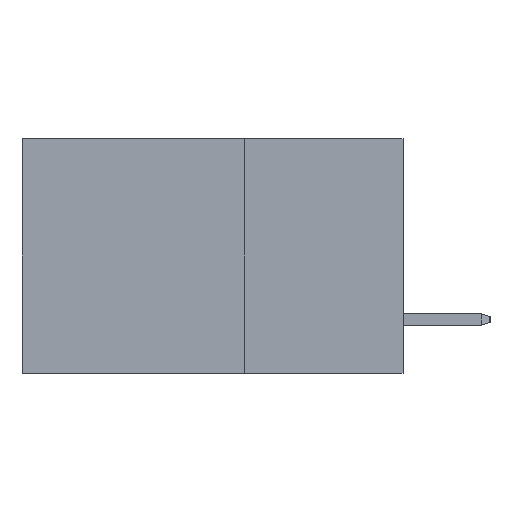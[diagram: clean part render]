
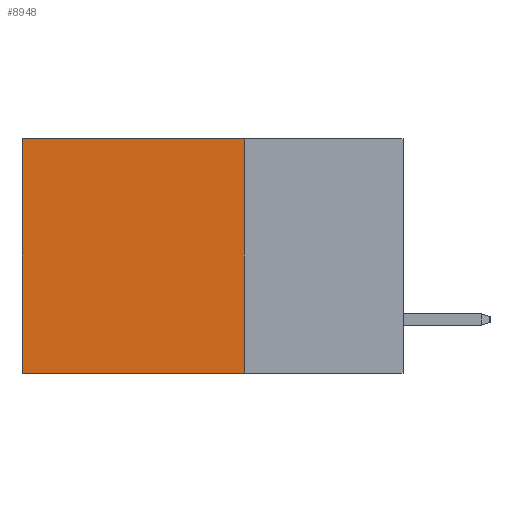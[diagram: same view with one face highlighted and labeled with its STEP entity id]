
A CAD part, left-side view. The second image highlights one B-rep face of the part: STEP entity #8948.
In plain terms, the highlighted planar face has unit normal (-1, 0, 0).
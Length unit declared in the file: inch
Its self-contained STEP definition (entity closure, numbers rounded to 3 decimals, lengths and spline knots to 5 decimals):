
#58 = PLANE ( 'NONE',  #7487 ) ;
#1327 = EDGE_LOOP ( 'NONE', ( #10557, #2436, #4083, #4589 ) ) ;
#2436 = ORIENTED_EDGE ( 'NONE', *, *, #5455, .F. ) ;
#2634 = CARTESIAN_POINT ( 'NONE',  ( 0.2875, 0.25, 0. ) ) ;
#2853 = CARTESIAN_POINT ( 'NONE',  ( 0.2875, 0.25, 0. ) ) ;
#3242 = DIRECTION ( 'NONE',  ( 0., 0., -1. ) ) ;
#3388 = DIRECTION ( 'NONE',  ( 0., 0., -1. ) ) ;
#3649 = VECTOR ( 'NONE', #3388, 39.37008 ) ;
#3777 = VERTEX_POINT ( 'NONE', #8731 ) ;
#4083 = ORIENTED_EDGE ( 'NONE', *, *, #8963, .F. ) ;
#4140 = CARTESIAN_POINT ( 'NONE',  ( 0.2875, 0.25, 0. ) ) ;
#4499 = VECTOR ( 'NONE', #8467, 39.37008 ) ;
#4589 = ORIENTED_EDGE ( 'NONE', *, *, #8456, .T. ) ;
#5147 = FACE_OUTER_BOUND ( 'NONE', #1327, .T. ) ;
#5455 = EDGE_CURVE ( 'NONE', #6212, #3777, #8843, .T. ) ;
#5502 = CARTESIAN_POINT ( 'NONE',  ( 0.2875, 0.6, 0. ) ) ;
#6212 = VERTEX_POINT ( 'NONE', #12421 ) ;
#6459 = DIRECTION ( 'NONE',  ( 1., 0., 0. ) ) ;
#6574 = DIRECTION ( 'NONE',  ( 0., 0., -1. ) ) ;
#7487 = AXIS2_PLACEMENT_3D ( 'NONE', #4140, #6459, #6574 ) ;
#7591 = LINE ( 'NONE', #9447, #4499 ) ;
#8167 = CARTESIAN_POINT ( 'NONE',  ( 0.2875, 0.6, 0. ) ) ;
#8456 = EDGE_CURVE ( 'NONE', #12430, #11397, #7591, .T. ) ;
#8467 = DIRECTION ( 'NONE',  ( 0., 1., 0. ) ) ;
#8696 = DIRECTION ( 'NONE',  ( 0., 1., 0. ) ) ;
#8731 = CARTESIAN_POINT ( 'NONE',  ( 0.2875, 0.6, -0.37 ) ) ;
#8843 = LINE ( 'NONE', #10886, #12473 ) ;
#8948 = ADVANCED_FACE ( 'NONE', ( #5147 ), #58, .F. ) ;
#8963 = EDGE_CURVE ( 'NONE', #12430, #6212, #12552, .T. ) ;
#9447 = CARTESIAN_POINT ( 'NONE',  ( 0.2875, 0.25, 0. ) ) ;
#10557 = ORIENTED_EDGE ( 'NONE', *, *, #11148, .T. ) ;
#10664 = VECTOR ( 'NONE', #3242, 39.37008 ) ;
#10886 = CARTESIAN_POINT ( 'NONE',  ( 0.2875, 0.25, -0.37 ) ) ;
#11148 = EDGE_CURVE ( 'NONE', #11397, #3777, #11527, .T. ) ;
#11397 = VERTEX_POINT ( 'NONE', #8167 ) ;
#11527 = LINE ( 'NONE', #5502, #10664 ) ;
#12421 = CARTESIAN_POINT ( 'NONE',  ( 0.2875, 0.25, -0.37 ) ) ;
#12430 = VERTEX_POINT ( 'NONE', #2853 ) ;
#12473 = VECTOR ( 'NONE', #8696, 39.37008 ) ;
#12552 = LINE ( 'NONE', #2634, #3649 ) ;
